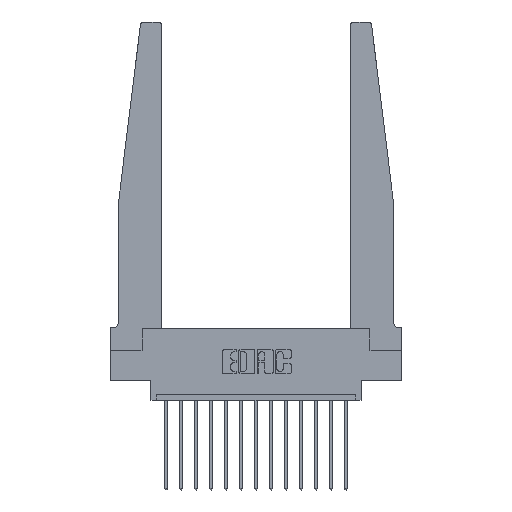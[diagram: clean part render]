
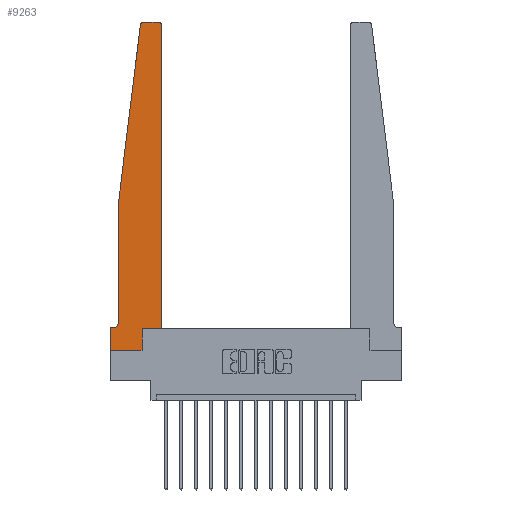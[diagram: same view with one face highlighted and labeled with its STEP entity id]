
A CAD part, top view. The second image highlights one B-rep face of the part: STEP entity #9263.
In plain terms, the highlighted planar face has unit normal (0, 0, 1).
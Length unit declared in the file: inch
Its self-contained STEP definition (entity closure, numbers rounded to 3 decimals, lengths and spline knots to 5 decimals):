
#19 = DIRECTION ( 'NONE',  ( 0., 0., 1. ) ) ;
#42 = ORIENTED_EDGE ( 'NONE', *, *, #1475, .T. ) ;
#77 = CARTESIAN_POINT ( 'NONE',  ( 0.065, 0.2375, 0.37 ) ) ;
#279 = LINE ( 'NONE', #13971, #14976 ) ;
#453 = DIRECTION ( 'NONE',  ( 0., -1., 0. ) ) ;
#601 = VECTOR ( 'NONE', #7230, 39.37008 ) ;
#943 = VERTEX_POINT ( 'NONE', #13438 ) ;
#1167 = DIRECTION ( 'NONE',  ( 0., -1., 0. ) ) ;
#1238 = CARTESIAN_POINT ( 'NONE',  ( 0.27653, 2.72, 0.37 ) ) ;
#1456 = ORIENTED_EDGE ( 'NONE', *, *, #11987, .T. ) ;
#1475 = EDGE_CURVE ( 'NONE', #10208, #8442, #14255, .T. ) ;
#1704 = AXIS2_PLACEMENT_3D ( 'NONE', #8846, #3521, #3570 ) ;
#1737 = CARTESIAN_POINT ( 'NONE',  ( 0.24675, 2.72367, 0.37 ) ) ;
#1757 = LINE ( 'NONE', #9835, #7649 ) ;
#1942 = AXIS2_PLACEMENT_3D ( 'NONE', #12021, #6868, #14729 ) ;
#2143 = CARTESIAN_POINT ( 'NONE',  ( 0., 0.1875, 0.37 ) ) ;
#2287 = VERTEX_POINT ( 'NONE', #3903 ) ;
#2621 = ORIENTED_EDGE ( 'NONE', *, *, #11668, .T. ) ;
#2874 = ORIENTED_EDGE ( 'NONE', *, *, #8815, .T. ) ;
#2875 = ORIENTED_EDGE ( 'NONE', *, *, #7706, .T. ) ;
#3162 = VERTEX_POINT ( 'NONE', #9297 ) ;
#3366 = EDGE_CURVE ( 'NONE', #10676, #3162, #1757, .T. ) ;
#3388 = VECTOR ( 'NONE', #453, 39.37008 ) ;
#3521 = DIRECTION ( 'NONE',  ( 0., 0., 1. ) ) ;
#3570 = DIRECTION ( 'NONE',  ( 1., 0., 0. ) ) ;
#3653 = CIRCLE ( 'NONE', #4742, 0.03 ) ;
#3903 = CARTESIAN_POINT ( 'NONE',  ( 0.065, 1.25, 0.37 ) ) ;
#4060 = EDGE_CURVE ( 'NONE', #3162, #13631, #14778, .T. ) ;
#4114 = CARTESIAN_POINT ( 'NONE',  ( 0.015, 0.1875, 0.37 ) ) ;
#4358 = EDGE_CURVE ( 'NONE', #2287, #7862, #12761, .T. ) ;
#4742 = AXIS2_PLACEMENT_3D ( 'NONE', #5217, #19, #9209 ) ;
#4796 = PLANE ( 'NONE',  #1704 ) ;
#4980 = VECTOR ( 'NONE', #1167, 39.37008 ) ;
#5217 = CARTESIAN_POINT ( 'NONE',  ( 0.395, 2.72, 0.37 ) ) ;
#5302 = LINE ( 'NONE', #13561, #601 ) ;
#5993 = LINE ( 'NONE', #16789, #4980 ) ;
#6562 = AXIS2_PLACEMENT_3D ( 'NONE', #1238, #16906, #11809 ) ;
#6574 = VECTOR ( 'NONE', #10773, 39.37008 ) ;
#6868 = DIRECTION ( 'NONE',  ( 0., 0., -1. ) ) ;
#7230 = DIRECTION ( 'NONE',  ( 0., 1., 0. ) ) ;
#7603 = LINE ( 'NONE', #13053, #6574 ) ;
#7649 = VECTOR ( 'NONE', #9819, 39.37008 ) ;
#7706 = EDGE_CURVE ( 'NONE', #14853, #9133, #5993, .T. ) ;
#7862 = VERTEX_POINT ( 'NONE', #77 ) ;
#8048 = CARTESIAN_POINT ( 'NONE',  ( 0.425, 0.18, 0.37 ) ) ;
#8061 = CARTESIAN_POINT ( 'NONE',  ( 0.065, 0.1875, 0.37 ) ) ;
#8078 = ORIENTED_EDGE ( 'NONE', *, *, #3366, .T. ) ;
#8267 = CARTESIAN_POINT ( 'NONE',  ( 0.065, 1.25, 0.37 ) ) ;
#8411 = ORIENTED_EDGE ( 'NONE', *, *, #13418, .T. ) ;
#8442 = VERTEX_POINT ( 'NONE', #12251 ) ;
#8815 = EDGE_CURVE ( 'NONE', #16676, #2287, #7603, .T. ) ;
#8846 = CARTESIAN_POINT ( 'NONE',  ( 0., 0.1875, 0.37 ) ) ;
#9121 = CARTESIAN_POINT ( 'NONE',  ( 0.425, 0.18, 0.37 ) ) ;
#9133 = VERTEX_POINT ( 'NONE', #13683 ) ;
#9209 = DIRECTION ( 'NONE',  ( 1., 0., 0. ) ) ;
#9263 = ADVANCED_FACE ( 'NONE', ( #11104 ), #4796, .T. ) ;
#9289 = ORIENTED_EDGE ( 'NONE', *, *, #12604, .T. ) ;
#9297 = CARTESIAN_POINT ( 'NONE',  ( 0.2605, 0.18, 0.37 ) ) ;
#9394 = DIRECTION ( 'NONE',  ( -1., 0., 0. ) ) ;
#9819 = DIRECTION ( 'NONE',  ( 0., 1., 0. ) ) ;
#9835 = CARTESIAN_POINT ( 'NONE',  ( 0.2605, 0.18, 0.37 ) ) ;
#9903 = VERTEX_POINT ( 'NONE', #4114 ) ;
#10208 = VERTEX_POINT ( 'NONE', #16341 ) ;
#10390 = DIRECTION ( 'NONE',  ( 1., 0., 0. ) ) ;
#10478 = DIRECTION ( 'NONE',  ( -1., 0., 0. ) ) ;
#10589 = VECTOR ( 'NONE', #10478, 39.37008 ) ;
#10630 = ORIENTED_EDGE ( 'NONE', *, *, #4060, .T. ) ;
#10676 = VERTEX_POINT ( 'NONE', #10745 ) ;
#10745 = CARTESIAN_POINT ( 'NONE',  ( 0.2605, 0., 0.37 ) ) ;
#10773 = DIRECTION ( 'NONE',  ( -0.122, -0.992, 0. ) ) ;
#10791 = CIRCLE ( 'NONE', #6562, 0.03 ) ;
#11104 = FACE_OUTER_BOUND ( 'NONE', #11825, .T. ) ;
#11668 = EDGE_CURVE ( 'NONE', #13631, #943, #5302, .T. ) ;
#11809 = DIRECTION ( 'NONE',  ( 1., 0., 0. ) ) ;
#11825 = EDGE_LOOP ( 'NONE', ( #42, #9289, #2874, #13636, #14270, #1456, #2875, #15133, #8078, #10630, #2621, #8411 ) ) ;
#11987 = EDGE_CURVE ( 'NONE', #9903, #14853, #15069, .T. ) ;
#12021 = CARTESIAN_POINT ( 'NONE',  ( 0.015, 0.2375, 0.37 ) ) ;
#12251 = CARTESIAN_POINT ( 'NONE',  ( 0.27653, 2.75, 0.37 ) ) ;
#12604 = EDGE_CURVE ( 'NONE', #8442, #16676, #10791, .T. ) ;
#12761 = LINE ( 'NONE', #8267, #3388 ) ;
#13053 = CARTESIAN_POINT ( 'NONE',  ( 0.065, 1.25, 0.37 ) ) ;
#13418 = EDGE_CURVE ( 'NONE', #943, #10208, #3653, .T. ) ;
#13438 = CARTESIAN_POINT ( 'NONE',  ( 0.425, 2.72, 0.37 ) ) ;
#13561 = CARTESIAN_POINT ( 'NONE',  ( 0.425, 0.18, 0.37 ) ) ;
#13631 = VERTEX_POINT ( 'NONE', #8048 ) ;
#13636 = ORIENTED_EDGE ( 'NONE', *, *, #4358, .T. ) ;
#13683 = CARTESIAN_POINT ( 'NONE',  ( 0., 0., 0.37 ) ) ;
#13726 = CIRCLE ( 'NONE', #1942, 0.05 ) ;
#13852 = VECTOR ( 'NONE', #9394, 39.37008 ) ;
#13971 = CARTESIAN_POINT ( 'NONE',  ( 0., 0., 0.37 ) ) ;
#14255 = LINE ( 'NONE', #16496, #10589 ) ;
#14270 = ORIENTED_EDGE ( 'NONE', *, *, #16533, .T. ) ;
#14729 = DIRECTION ( 'NONE',  ( -1., 0., 0. ) ) ;
#14778 = LINE ( 'NONE', #9121, #16828 ) ;
#14853 = VERTEX_POINT ( 'NONE', #2143 ) ;
#14976 = VECTOR ( 'NONE', #15361, 39.37008 ) ;
#15069 = LINE ( 'NONE', #8061, #13852 ) ;
#15133 = ORIENTED_EDGE ( 'NONE', *, *, #15667, .T. ) ;
#15361 = DIRECTION ( 'NONE',  ( 1., 0., 0. ) ) ;
#15667 = EDGE_CURVE ( 'NONE', #9133, #10676, #279, .T. ) ;
#16341 = CARTESIAN_POINT ( 'NONE',  ( 0.395, 2.75, 0.37 ) ) ;
#16496 = CARTESIAN_POINT ( 'NONE',  ( 0.25, 2.75, 0.37 ) ) ;
#16533 = EDGE_CURVE ( 'NONE', #7862, #9903, #13726, .T. ) ;
#16676 = VERTEX_POINT ( 'NONE', #1737 ) ;
#16789 = CARTESIAN_POINT ( 'NONE',  ( 0., 0., 0.37 ) ) ;
#16828 = VECTOR ( 'NONE', #10390, 39.37008 ) ;
#16906 = DIRECTION ( 'NONE',  ( 0., 0., 1. ) ) ;
